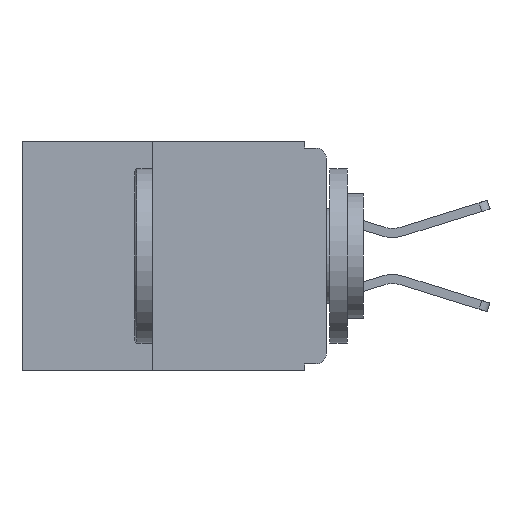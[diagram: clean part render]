
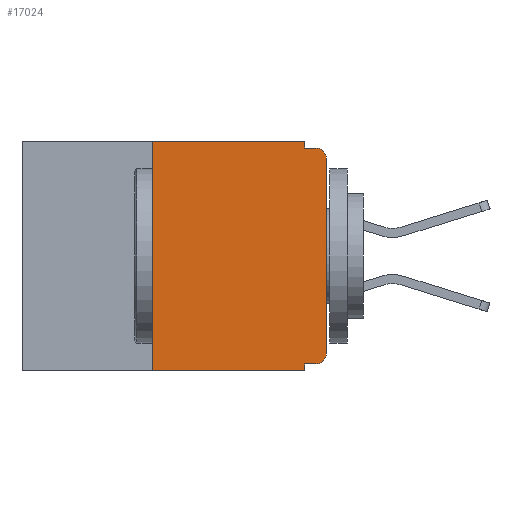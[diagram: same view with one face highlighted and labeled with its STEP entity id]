
A CAD part, left-side view. The second image highlights one B-rep face of the part: STEP entity #17024.
In plain terms, the highlighted planar face has unit normal (-1, 0, 0).
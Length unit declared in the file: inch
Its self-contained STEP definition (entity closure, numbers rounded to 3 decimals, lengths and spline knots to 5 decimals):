
#85 = LINE ( 'NONE', #1510, #13192 ) ;
#258 = CARTESIAN_POINT ( 'NONE',  ( 0., 0.437, 0. ) ) ;
#482 = CIRCLE ( 'NONE', #11516, 0.015 ) ;
#860 = AXIS2_PLACEMENT_3D ( 'NONE', #258, #18945, #8968 ) ;
#1084 = EDGE_CURVE ( 'NONE', #10571, #7379, #7552, .T. ) ;
#1150 = CARTESIAN_POINT ( 'NONE',  ( 0., 0.031, 0. ) ) ;
#1510 = CARTESIAN_POINT ( 'NONE',  ( 0., 0., -0.01 ) ) ;
#1943 = CIRCLE ( 'NONE', #5908, 0.015 ) ;
#2710 = VECTOR ( 'NONE', #15551, 39.37008 ) ;
#3634 = EDGE_LOOP ( 'NONE', ( #16100, #14804, #17421, #14109, #21601, #15455, #11976, #18005, #15176, #7547 ) ) ;
#3753 = CARTESIAN_POINT ( 'NONE',  ( 0., 0.031, -0.01 ) ) ;
#3764 = PLANE ( 'NONE',  #860 ) ;
#3913 = CARTESIAN_POINT ( 'NONE',  ( 0., 0.015, -0.305 ) ) ;
#4701 = CARTESIAN_POINT ( 'NONE',  ( 0., 0.031, -0.32 ) ) ;
#5013 = VECTOR ( 'NONE', #5775, 39.37008 ) ;
#5541 = LINE ( 'NONE', #12543, #5013 ) ;
#5624 = DIRECTION ( 'NONE',  ( 0., 0., -1. ) ) ;
#5764 = CARTESIAN_POINT ( 'NONE',  ( 0., 0.031, -0.33 ) ) ;
#5775 = DIRECTION ( 'NONE',  ( 0., 0., -1. ) ) ;
#5908 = AXIS2_PLACEMENT_3D ( 'NONE', #19251, #9264, #20886 ) ;
#6895 = DIRECTION ( 'NONE',  ( 0., 0., 1. ) ) ;
#7027 = VECTOR ( 'NONE', #18994, 39.37008 ) ;
#7060 = CARTESIAN_POINT ( 'NONE',  ( 0., 0.015, -0.01 ) ) ;
#7354 = CARTESIAN_POINT ( 'NONE',  ( 0., 0.25, 0. ) ) ;
#7379 = VERTEX_POINT ( 'NONE', #1150 ) ;
#7547 = ORIENTED_EDGE ( 'NONE', *, *, #19833, .T. ) ;
#7552 = LINE ( 'NONE', #18961, #7027 ) ;
#8437 = EDGE_CURVE ( 'NONE', #12997, #10900, #10129, .T. ) ;
#8968 = DIRECTION ( 'NONE',  ( 0., 0., -1. ) ) ;
#9155 = LINE ( 'NONE', #16971, #13598 ) ;
#9264 = DIRECTION ( 'NONE',  ( -1., 0., 0. ) ) ;
#10059 = DIRECTION ( 'NONE',  ( 0., -1., 0. ) ) ;
#10129 = LINE ( 'NONE', #18815, #13518 ) ;
#10310 = EDGE_CURVE ( 'NONE', #12332, #21572, #85, .T. ) ;
#10571 = VERTEX_POINT ( 'NONE', #7354 ) ;
#10900 = VERTEX_POINT ( 'NONE', #4701 ) ;
#11476 = EDGE_CURVE ( 'NONE', #7379, #12332, #19638, .T. ) ;
#11516 = AXIS2_PLACEMENT_3D ( 'NONE', #3913, #15769, #5624 ) ;
#11669 = CARTESIAN_POINT ( 'NONE',  ( 0., 0., -0.025 ) ) ;
#11976 = ORIENTED_EDGE ( 'NONE', *, *, #18371, .T. ) ;
#12320 = EDGE_CURVE ( 'NONE', #18062, #10571, #20628, .T. ) ;
#12332 = VERTEX_POINT ( 'NONE', #3753 ) ;
#12543 = CARTESIAN_POINT ( 'NONE',  ( 0., 0.031, -0.33 ) ) ;
#12997 = VERTEX_POINT ( 'NONE', #15737 ) ;
#13192 = VECTOR ( 'NONE', #10059, 39.37008 ) ;
#13518 = VECTOR ( 'NONE', #18791, 39.37008 ) ;
#13598 = VECTOR ( 'NONE', #6895, 39.37008 ) ;
#13802 = VERTEX_POINT ( 'NONE', #5764 ) ;
#13926 = CARTESIAN_POINT ( 'NONE',  ( 0., 0.25, -0.33 ) ) ;
#14109 = ORIENTED_EDGE ( 'NONE', *, *, #11476, .F. ) ;
#14804 = ORIENTED_EDGE ( 'NONE', *, *, #15103, .T. ) ;
#15103 = EDGE_CURVE ( 'NONE', #15409, #21572, #1943, .T. ) ;
#15176 = ORIENTED_EDGE ( 'NONE', *, *, #8437, .F. ) ;
#15259 = VECTOR ( 'NONE', #19678, 39.37008 ) ;
#15409 = VERTEX_POINT ( 'NONE', #11669 ) ;
#15455 = ORIENTED_EDGE ( 'NONE', *, *, #12320, .F. ) ;
#15551 = DIRECTION ( 'NONE',  ( 0., 0., 1. ) ) ;
#15737 = CARTESIAN_POINT ( 'NONE',  ( 0., 0.015, -0.32 ) ) ;
#15769 = DIRECTION ( 'NONE',  ( -1., 0., 0. ) ) ;
#16100 = ORIENTED_EDGE ( 'NONE', *, *, #16249, .T. ) ;
#16249 = EDGE_CURVE ( 'NONE', #20834, #15409, #9155, .T. ) ;
#16369 = CARTESIAN_POINT ( 'NONE',  ( 0., 0.031, 0. ) ) ;
#16971 = CARTESIAN_POINT ( 'NONE',  ( 0., 0., 0. ) ) ;
#17024 = ADVANCED_FACE ( 'NONE', ( #20560 ), #3764, .F. ) ;
#17421 = ORIENTED_EDGE ( 'NONE', *, *, #10310, .F. ) ;
#17523 = CARTESIAN_POINT ( 'NONE',  ( 0., 0.437, -0.33 ) ) ;
#18005 = ORIENTED_EDGE ( 'NONE', *, *, #21122, .F. ) ;
#18062 = VERTEX_POINT ( 'NONE', #21609 ) ;
#18371 = EDGE_CURVE ( 'NONE', #18062, #13802, #21513, .T. ) ;
#18791 = DIRECTION ( 'NONE',  ( 0., 1., 0. ) ) ;
#18815 = CARTESIAN_POINT ( 'NONE',  ( 0., 0., -0.32 ) ) ;
#18945 = DIRECTION ( 'NONE',  ( 1., 0., 0. ) ) ;
#18961 = CARTESIAN_POINT ( 'NONE',  ( 0., 0.437, 0. ) ) ;
#18994 = DIRECTION ( 'NONE',  ( 0., -1., 0. ) ) ;
#19171 = DIRECTION ( 'NONE',  ( 0., -1., 0. ) ) ;
#19251 = CARTESIAN_POINT ( 'NONE',  ( 0., 0.015, -0.025 ) ) ;
#19638 = LINE ( 'NONE', #16369, #15259 ) ;
#19678 = DIRECTION ( 'NONE',  ( 0., 0., -1. ) ) ;
#19833 = EDGE_CURVE ( 'NONE', #12997, #20834, #482, .T. ) ;
#19990 = VECTOR ( 'NONE', #19171, 39.37008 ) ;
#20560 = FACE_OUTER_BOUND ( 'NONE', #3634, .T. ) ;
#20628 = LINE ( 'NONE', #13926, #2710 ) ;
#20834 = VERTEX_POINT ( 'NONE', #21686 ) ;
#20886 = DIRECTION ( 'NONE',  ( 0., 0., -1. ) ) ;
#21122 = EDGE_CURVE ( 'NONE', #10900, #13802, #5541, .T. ) ;
#21513 = LINE ( 'NONE', #17523, #19990 ) ;
#21572 = VERTEX_POINT ( 'NONE', #7060 ) ;
#21601 = ORIENTED_EDGE ( 'NONE', *, *, #1084, .F. ) ;
#21609 = CARTESIAN_POINT ( 'NONE',  ( 0., 0.25, -0.33 ) ) ;
#21686 = CARTESIAN_POINT ( 'NONE',  ( 0., 0., -0.305 ) ) ;
